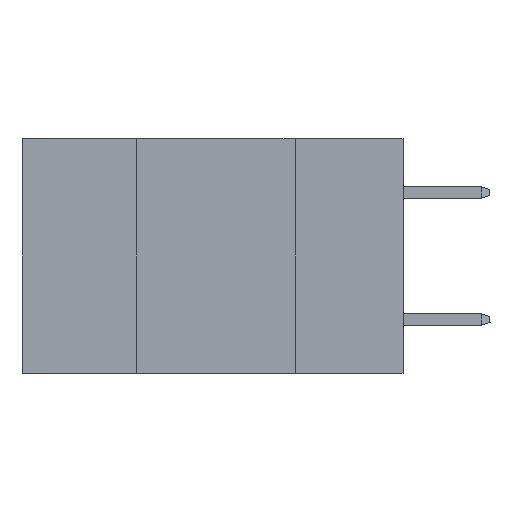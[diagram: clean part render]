
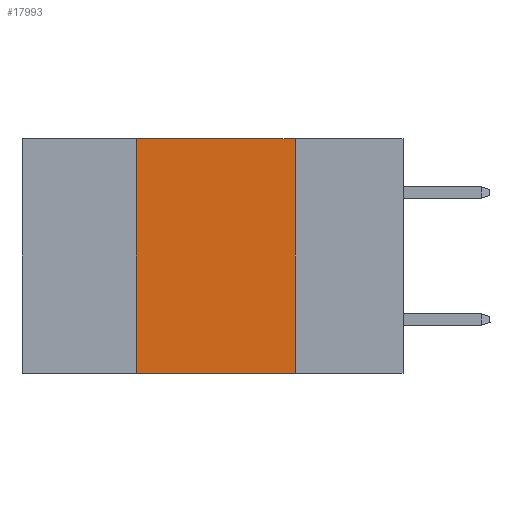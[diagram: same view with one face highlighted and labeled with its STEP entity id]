
A CAD part, left-side view. The second image highlights one B-rep face of the part: STEP entity #17993.
In plain terms, the highlighted planar face has unit normal (-1, 0, 0).
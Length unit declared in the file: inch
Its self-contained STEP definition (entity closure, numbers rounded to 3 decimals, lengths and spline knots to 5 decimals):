
#313 = VERTEX_POINT ( 'NONE', #19925 ) ;
#452 = LINE ( 'NONE', #14845, #24583 ) ;
#548 = CARTESIAN_POINT ( 'NONE',  ( 0., 0.17, -0.37 ) ) ;
#1151 = EDGE_CURVE ( 'NONE', #11596, #2816, #452, .T. ) ;
#2022 = ORIENTED_EDGE ( 'NONE', *, *, #11938, .F. ) ;
#2645 = EDGE_CURVE ( 'NONE', #11021, #2816, #20130, .T. ) ;
#2816 = VERTEX_POINT ( 'NONE', #548 ) ;
#4000 = VECTOR ( 'NONE', #19780, 39.37008 ) ;
#7309 = LINE ( 'NONE', #7707, #4000 ) ;
#7358 = CARTESIAN_POINT ( 'NONE',  ( 0., 0.42, -0.37 ) ) ;
#7707 = CARTESIAN_POINT ( 'NONE',  ( 0., 0.6, 0. ) ) ;
#8483 = DIRECTION ( 'NONE',  ( 0., 0., -1. ) ) ;
#9425 = CARTESIAN_POINT ( 'NONE',  ( 0., 0.42, 0. ) ) ;
#9432 = ORIENTED_EDGE ( 'NONE', *, *, #1151, .F. ) ;
#9740 = VECTOR ( 'NONE', #26489, 39.37008 ) ;
#11021 = VERTEX_POINT ( 'NONE', #7358 ) ;
#11596 = VERTEX_POINT ( 'NONE', #26286 ) ;
#11938 = EDGE_CURVE ( 'NONE', #11021, #313, #19746, .T. ) ;
#14845 = CARTESIAN_POINT ( 'NONE',  ( 0., 0.17, 0. ) ) ;
#15110 = FACE_OUTER_BOUND ( 'NONE', #20132, .T. ) ;
#16362 = DIRECTION ( 'NONE',  ( 0., 0., 1. ) ) ;
#16758 = CARTESIAN_POINT ( 'NONE',  ( 0., 0.6, 0. ) ) ;
#16813 = ORIENTED_EDGE ( 'NONE', *, *, #2645, .T. ) ;
#17464 = ORIENTED_EDGE ( 'NONE', *, *, #23546, .F. ) ;
#17993 = ADVANCED_FACE ( 'NONE', ( #15110 ), #18802, .F. ) ;
#18802 = PLANE ( 'NONE',  #26510 ) ;
#19746 = LINE ( 'NONE', #9425, #24020 ) ;
#19780 = DIRECTION ( 'NONE',  ( 0., -1., 0. ) ) ;
#19925 = CARTESIAN_POINT ( 'NONE',  ( 0., 0.42, 0. ) ) ;
#20130 = LINE ( 'NONE', #22689, #9740 ) ;
#20132 = EDGE_LOOP ( 'NONE', ( #9432, #17464, #2022, #16813 ) ) ;
#21359 = DIRECTION ( 'NONE',  ( 1., 0., 0. ) ) ;
#22689 = CARTESIAN_POINT ( 'NONE',  ( 0., 0.6, -0.37 ) ) ;
#22716 = DIRECTION ( 'NONE',  ( 0., 0., -1. ) ) ;
#23546 = EDGE_CURVE ( 'NONE', #313, #11596, #7309, .T. ) ;
#24020 = VECTOR ( 'NONE', #16362, 39.37008 ) ;
#24583 = VECTOR ( 'NONE', #22716, 39.37008 ) ;
#26286 = CARTESIAN_POINT ( 'NONE',  ( 0., 0.17, 0. ) ) ;
#26489 = DIRECTION ( 'NONE',  ( 0., -1., 0. ) ) ;
#26510 = AXIS2_PLACEMENT_3D ( 'NONE', #16758, #21359, #8483 ) ;
